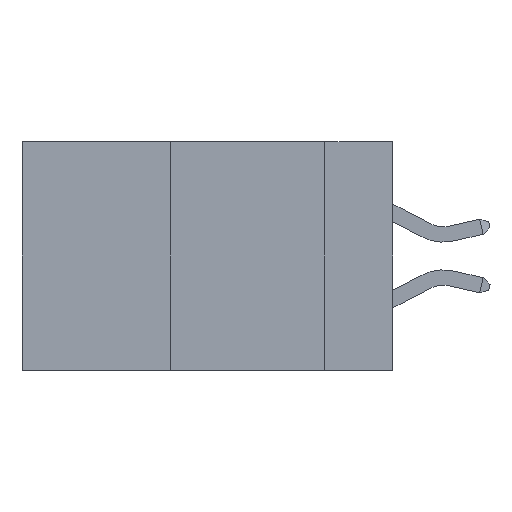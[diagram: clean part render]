
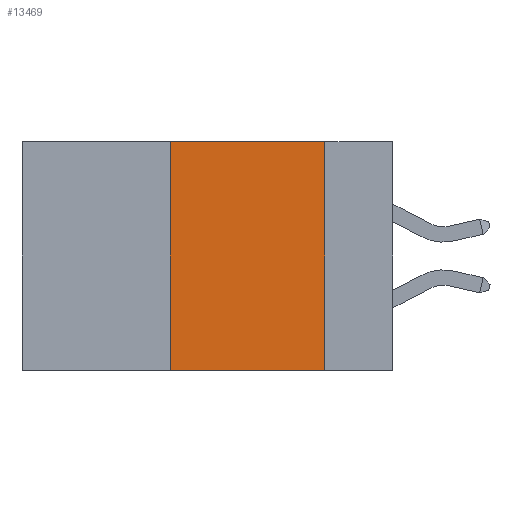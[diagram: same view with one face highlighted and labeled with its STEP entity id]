
A CAD part, left-side view. The second image highlights one B-rep face of the part: STEP entity #13469.
In plain terms, the highlighted planar face has unit normal (-1, 0, 0).
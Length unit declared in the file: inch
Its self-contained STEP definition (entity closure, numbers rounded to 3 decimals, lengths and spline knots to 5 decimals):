
#766 = LINE ( 'NONE', #20316, #10070 ) ;
#918 = LINE ( 'NONE', #17862, #10214 ) ;
#1739 = EDGE_LOOP ( 'NONE', ( #2901, #8992, #14288, #10135 ) ) ;
#1750 = EDGE_CURVE ( 'NONE', #17581, #14564, #22570, .T. ) ;
#2309 = AXIS2_PLACEMENT_3D ( 'NONE', #8528, #13874, #2995 ) ;
#2901 = ORIENTED_EDGE ( 'NONE', *, *, #13377, .F. ) ;
#2907 = PLANE ( 'NONE',  #2309 ) ;
#2995 = DIRECTION ( 'NONE',  ( 0., 0., -1. ) ) ;
#7846 = DIRECTION ( 'NONE',  ( 0., -1., 0. ) ) ;
#8528 = CARTESIAN_POINT ( 'NONE',  ( 0., 0.6, 0. ) ) ;
#8929 = FACE_OUTER_BOUND ( 'NONE', #1739, .T. ) ;
#8992 = ORIENTED_EDGE ( 'NONE', *, *, #1750, .F. ) ;
#10070 = VECTOR ( 'NONE', #11977, 39.37008 ) ;
#10135 = ORIENTED_EDGE ( 'NONE', *, *, #11535, .T. ) ;
#10214 = VECTOR ( 'NONE', #19474, 39.37008 ) ;
#11535 = EDGE_CURVE ( 'NONE', #16829, #17228, #918, .T. ) ;
#11977 = DIRECTION ( 'NONE',  ( 0., 0., -1. ) ) ;
#12878 = CARTESIAN_POINT ( 'NONE',  ( 0., 0.11, -0.37 ) ) ;
#13377 = EDGE_CURVE ( 'NONE', #14564, #17228, #766, .T. ) ;
#13469 = ADVANCED_FACE ( 'NONE', ( #8929 ), #2907, .F. ) ;
#13598 = VECTOR ( 'NONE', #22652, 39.37008 ) ;
#13784 = VECTOR ( 'NONE', #7846, 39.37008 ) ;
#13874 = DIRECTION ( 'NONE',  ( 1., 0., 0. ) ) ;
#14151 = CARTESIAN_POINT ( 'NONE',  ( 0., 0.11, 0. ) ) ;
#14152 = EDGE_CURVE ( 'NONE', #16829, #17581, #14183, .T. ) ;
#14183 = LINE ( 'NONE', #19375, #13598 ) ;
#14288 = ORIENTED_EDGE ( 'NONE', *, *, #14152, .F. ) ;
#14564 = VERTEX_POINT ( 'NONE', #14151 ) ;
#15516 = CARTESIAN_POINT ( 'NONE',  ( 0., 0.36, -0.37 ) ) ;
#16829 = VERTEX_POINT ( 'NONE', #15516 ) ;
#17228 = VERTEX_POINT ( 'NONE', #12878 ) ;
#17581 = VERTEX_POINT ( 'NONE', #18689 ) ;
#17862 = CARTESIAN_POINT ( 'NONE',  ( 0., 0.6, -0.37 ) ) ;
#18689 = CARTESIAN_POINT ( 'NONE',  ( 0., 0.36, 0. ) ) ;
#19375 = CARTESIAN_POINT ( 'NONE',  ( 0., 0.36, 0. ) ) ;
#19474 = DIRECTION ( 'NONE',  ( 0., -1., 0. ) ) ;
#20316 = CARTESIAN_POINT ( 'NONE',  ( 0., 0.11, 0. ) ) ;
#21399 = CARTESIAN_POINT ( 'NONE',  ( 0., 0.6, 0. ) ) ;
#22570 = LINE ( 'NONE', #21399, #13784 ) ;
#22652 = DIRECTION ( 'NONE',  ( 0., 0., 1. ) ) ;
